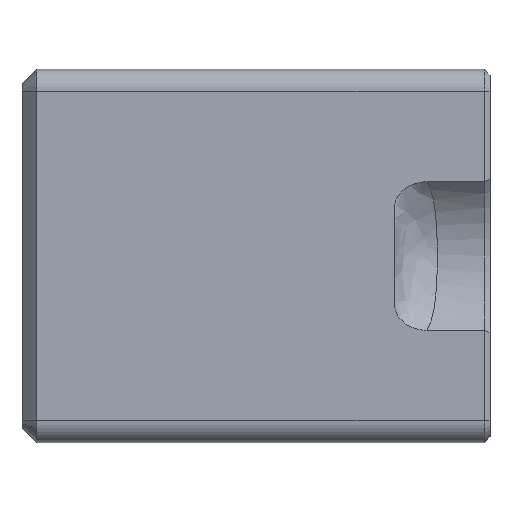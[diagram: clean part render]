
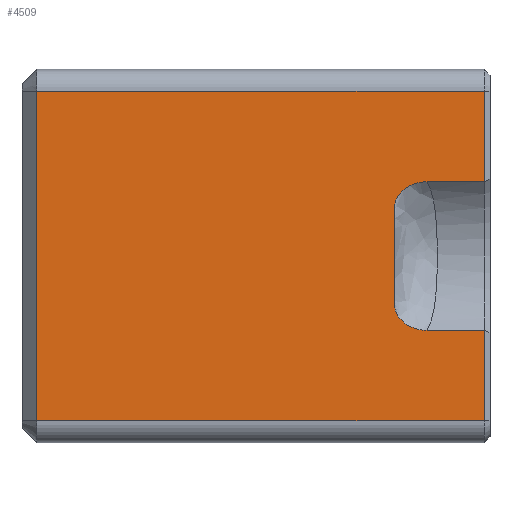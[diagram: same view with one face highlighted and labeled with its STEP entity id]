
A CAD part, front view. The second image highlights one B-rep face of the part: STEP entity #4509.
In plain terms, the highlighted planar face has unit normal (0, -1, 0).
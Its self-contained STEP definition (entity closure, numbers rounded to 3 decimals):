
#543=B_SPLINE_CURVE_WITH_KNOTS('',3,(#12359,#12360,#12361,#12362,#12363,
#12364,#12365,#12366,#12367,#12368,#12369,#12370,#12371,#12372,#12373,#12374,
#12375,#12376,#12377,#12378),.UNSPECIFIED.,.F.,.F.,(4,2,2,2,2,2,2,2,2,4),
(0.,0.,0.,0.002,0.007,
0.018,0.04,0.085,0.157,
0.234),.UNSPECIFIED.);
#544=B_SPLINE_CURVE_WITH_KNOTS('',3,(#12382,#12383,#12384,#12385,#12386,
#12387,#12388,#12389,#12390,#12391,#12392,#12393,#12394,#12395,#12396,#12397,
#12398,#12399,#12400,#12401),.UNSPECIFIED.,.F.,.F.,(4,2,2,2,2,2,2,2,2,4),
(0.,0.102,0.197,0.257,0.286,
0.3,0.306,0.31,0.31,
0.31),.UNSPECIFIED.);
#610=PLANE('',#4834);
#937=FACE_OUTER_BOUND('',#1213,.T.);
#1213=EDGE_LOOP('',(#4151,#4152,#4153,#4154,#4155,#4156,#4157,#4158,#4159,
#4160));
#1355=LINE('',#12326,#1508);
#1364=LINE('',#12348,#1517);
#1365=LINE('',#12353,#1518);
#1366=LINE('',#12357,#1519);
#1367=LINE('',#12380,#1520);
#1368=LINE('',#12402,#1521);
#1369=LINE('',#12404,#1522);
#1370=LINE('',#12405,#1523);
#1508=VECTOR('',#5513,10.);
#1517=VECTOR('',#5546,10.);
#1518=VECTOR('',#5553,10.);
#1519=VECTOR('',#5558,10.);
#1520=VECTOR('',#5559,10.);
#1521=VECTOR('',#5560,10.);
#1522=VECTOR('',#5561,10.);
#1523=VECTOR('',#5562,10.);
#2113=VERTEX_POINT('',#12313);
#2114=VERTEX_POINT('',#12318);
#2115=VERTEX_POINT('',#12325);
#2116=VERTEX_POINT('',#12344);
#2117=VERTEX_POINT('',#12352);
#2118=VERTEX_POINT('',#12356);
#2119=VERTEX_POINT('',#12358);
#2120=VERTEX_POINT('',#12379);
#2121=VERTEX_POINT('',#12381);
#2122=VERTEX_POINT('',#12403);
#2788=EDGE_CURVE('',#2114,#2115,#1355,.T.);
#2801=EDGE_CURVE('',#2116,#2113,#1364,.T.);
#2803=EDGE_CURVE('',#2115,#2117,#1365,.T.);
#2805=EDGE_CURVE('',#2114,#2118,#1366,.T.);
#2806=EDGE_CURVE('',#2119,#2118,#543,.T.);
#2807=EDGE_CURVE('',#2119,#2120,#1367,.T.);
#2808=EDGE_CURVE('',#2120,#2121,#544,.F.);
#2809=EDGE_CURVE('',#2121,#2113,#1368,.T.);
#2810=EDGE_CURVE('',#2122,#2116,#1369,.T.);
#2811=EDGE_CURVE('',#2117,#2122,#1370,.T.);
#4151=ORIENTED_EDGE('',*,*,#2788,.F.);
#4152=ORIENTED_EDGE('',*,*,#2805,.T.);
#4153=ORIENTED_EDGE('',*,*,#2806,.F.);
#4154=ORIENTED_EDGE('',*,*,#2807,.T.);
#4155=ORIENTED_EDGE('',*,*,#2808,.T.);
#4156=ORIENTED_EDGE('',*,*,#2809,.T.);
#4157=ORIENTED_EDGE('',*,*,#2801,.F.);
#4158=ORIENTED_EDGE('',*,*,#2810,.F.);
#4159=ORIENTED_EDGE('',*,*,#2811,.F.);
#4160=ORIENTED_EDGE('',*,*,#2803,.F.);
#4509=ADVANCED_FACE('',(#937),#610,.T.);
#4834=AXIS2_PLACEMENT_3D('',#12355,#5556,#5557);
#5513=DIRECTION('',(0.,0.,-1.));
#5546=DIRECTION('',(0.,0.,-1.));
#5553=DIRECTION('',(-1.,0.,0.));
#5556=DIRECTION('center_axis',(0.,-1.,0.));
#5557=DIRECTION('ref_axis',(0.,0.,1.));
#5558=DIRECTION('',(-1.,0.,0.));
#5559=DIRECTION('',(0.,0.,1.));
#5560=DIRECTION('',(1.,0.,0.));
#5561=DIRECTION('',(1.,0.,0.));
#5562=DIRECTION('',(0.,0.,1.));
#12313=CARTESIAN_POINT('',(-183.534,-11.455,5.083));
#12318=CARTESIAN_POINT('',(-183.534,-11.455,-5.083));
#12325=CARTESIAN_POINT('',(-183.534,-11.455,-11.264));
#12326=CARTESIAN_POINT('',(-183.534,-11.455,-6.128));
#12344=CARTESIAN_POINT('',(-183.534,-11.455,11.264));
#12348=CARTESIAN_POINT('',(-183.534,-11.455,-6.128));
#12352=CARTESIAN_POINT('',(-214.134,-11.455,-11.264));
#12353=CARTESIAN_POINT('',(-183.134,-11.455,-11.264));
#12355=CARTESIAN_POINT('Origin',(-183.134,-11.455,-12.256));
#12356=CARTESIAN_POINT('',(-187.44,-11.455,-5.083));
#12357=CARTESIAN_POINT('',(-183.134,-11.455,-5.083));
#12358=CARTESIAN_POINT('',(-189.634,-11.455,-3.546));
#12359=CARTESIAN_POINT('Ctrl Pts',(-189.634,-11.455,-3.546));
#12360=CARTESIAN_POINT('Ctrl Pts',(-189.634,-11.455,-3.546));
#12361=CARTESIAN_POINT('Ctrl Pts',(-189.634,-11.455,-3.547));
#12362=CARTESIAN_POINT('Ctrl Pts',(-189.634,-11.455,-3.548));
#12363=CARTESIAN_POINT('Ctrl Pts',(-189.634,-11.455,-3.549));
#12364=CARTESIAN_POINT('Ctrl Pts',(-189.634,-11.455,-3.558));
#12365=CARTESIAN_POINT('Ctrl Pts',(-189.633,-11.455,-3.566));
#12366=CARTESIAN_POINT('Ctrl Pts',(-189.63,-11.455,-3.592));
#12367=CARTESIAN_POINT('Ctrl Pts',(-189.627,-11.455,-3.61));
#12368=CARTESIAN_POINT('Ctrl Pts',(-189.616,-11.455,-3.667));
#12369=CARTESIAN_POINT('Ctrl Pts',(-189.605,-11.455,-3.707));
#12370=CARTESIAN_POINT('Ctrl Pts',(-189.566,-11.455,-3.826));
#12371=CARTESIAN_POINT('Ctrl Pts',(-189.531,-11.455,-3.905));
#12372=CARTESIAN_POINT('Ctrl Pts',(-189.407,-11.455,-4.136));
#12373=CARTESIAN_POINT('Ctrl Pts',(-189.297,-11.455,
-4.279));
#12374=CARTESIAN_POINT('Ctrl Pts',(-188.973,-11.455,
-4.603));
#12375=CARTESIAN_POINT('Ctrl Pts',(-188.724,-11.455,-4.771));
#12376=CARTESIAN_POINT('Ctrl Pts',(-188.119,-11.455,-5.02));
#12377=CARTESIAN_POINT('Ctrl Pts',(-187.781,-11.455,-5.083));
#12378=CARTESIAN_POINT('Ctrl Pts',(-187.44,-11.455,-5.083));
#12379=CARTESIAN_POINT('',(-189.634,-11.455,3.546));
#12380=CARTESIAN_POINT('',(-189.634,-11.455,-6.128));
#12381=CARTESIAN_POINT('',(-187.44,-11.455,5.083));
#12382=CARTESIAN_POINT('Ctrl Pts',(-187.44,-11.455,5.083));
#12383=CARTESIAN_POINT('Ctrl Pts',(-187.781,-11.455,5.083));
#12384=CARTESIAN_POINT('Ctrl Pts',(-188.119,-11.455,5.02));
#12385=CARTESIAN_POINT('Ctrl Pts',(-188.724,-11.455,4.771));
#12386=CARTESIAN_POINT('Ctrl Pts',(-188.973,-11.455,
4.603));
#12387=CARTESIAN_POINT('Ctrl Pts',(-189.297,-11.455,
4.279));
#12388=CARTESIAN_POINT('Ctrl Pts',(-189.407,-11.455,4.136));
#12389=CARTESIAN_POINT('Ctrl Pts',(-189.531,-11.455,3.905));
#12390=CARTESIAN_POINT('Ctrl Pts',(-189.566,-11.455,3.826));
#12391=CARTESIAN_POINT('Ctrl Pts',(-189.605,-11.455,3.707));
#12392=CARTESIAN_POINT('Ctrl Pts',(-189.616,-11.455,3.667));
#12393=CARTESIAN_POINT('Ctrl Pts',(-189.627,-11.455,3.61));
#12394=CARTESIAN_POINT('Ctrl Pts',(-189.63,-11.455,3.592));
#12395=CARTESIAN_POINT('Ctrl Pts',(-189.633,-11.455,3.565));
#12396=CARTESIAN_POINT('Ctrl Pts',(-189.634,-11.455,3.557));
#12397=CARTESIAN_POINT('Ctrl Pts',(-189.634,-11.455,3.549));
#12398=CARTESIAN_POINT('Ctrl Pts',(-189.634,-11.455,3.548));
#12399=CARTESIAN_POINT('Ctrl Pts',(-189.634,-11.455,3.547));
#12400=CARTESIAN_POINT('Ctrl Pts',(-189.634,-11.455,3.546));
#12401=CARTESIAN_POINT('Ctrl Pts',(-189.634,-11.455,3.546));
#12402=CARTESIAN_POINT('',(-183.134,-11.455,5.083));
#12403=CARTESIAN_POINT('',(-214.134,-11.455,11.264));
#12404=CARTESIAN_POINT('',(-183.134,-11.455,11.264));
#12405=CARTESIAN_POINT('',(-214.134,-11.455,-6.128));
